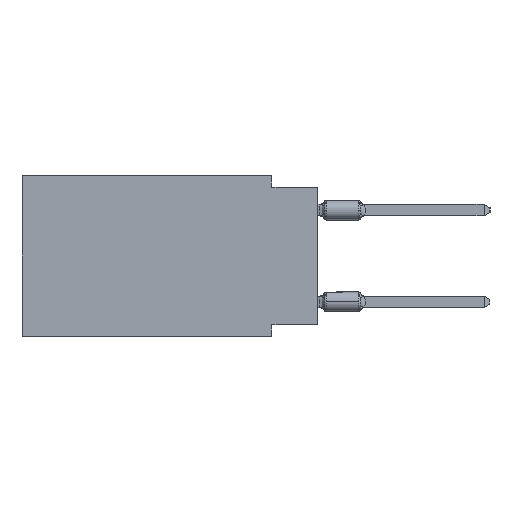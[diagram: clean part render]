
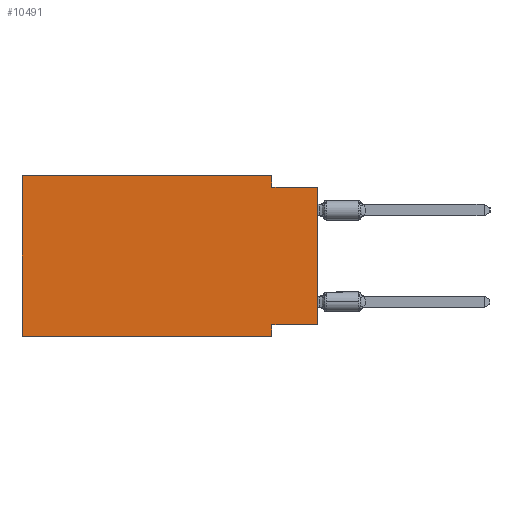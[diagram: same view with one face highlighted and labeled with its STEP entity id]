
A CAD part, left-side view. The second image highlights one B-rep face of the part: STEP entity #10491.
In plain terms, the highlighted planar face has unit normal (-1, 0, 0).
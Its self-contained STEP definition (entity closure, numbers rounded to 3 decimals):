
#1239 = CARTESIAN_POINT ( 'NONE',  ( 0., 16.383, 0. ) ) ;
#2220 = DIRECTION ( 'NONE',  ( 0., 0., 1. ) ) ;
#2269 = CARTESIAN_POINT ( 'NONE',  ( 0., 2.54, -0.635 ) ) ;
#2638 = ORIENTED_EDGE ( 'NONE', *, *, #15084, .T. ) ;
#2737 = LINE ( 'NONE', #10345, #23848 ) ;
#2896 = EDGE_CURVE ( 'NONE', #24381, #5201, #14568, .T. ) ;
#3232 = LINE ( 'NONE', #1239, #19793 ) ;
#3311 = CARTESIAN_POINT ( 'NONE',  ( 0., 0., -0.635 ) ) ;
#3857 = CARTESIAN_POINT ( 'NONE',  ( 0., 16.383, 0. ) ) ;
#4257 = EDGE_CURVE ( 'NONE', #8204, #5927, #3232, .T. ) ;
#4391 = EDGE_CURVE ( 'NONE', #21797, #8204, #22811, .T. ) ;
#4645 = VECTOR ( 'NONE', #2220, 1000. ) ;
#5201 = VERTEX_POINT ( 'NONE', #11739 ) ;
#5256 = PLANE ( 'NONE',  #18467 ) ;
#5927 = VERTEX_POINT ( 'NONE', #16566 ) ;
#5961 = CARTESIAN_POINT ( 'NONE',  ( 0., 0., 0. ) ) ;
#6499 = EDGE_CURVE ( 'NONE', #5201, #7645, #16034, .T. ) ;
#6882 = CARTESIAN_POINT ( 'NONE',  ( 0., 0., -0.635 ) ) ;
#7252 = CARTESIAN_POINT ( 'NONE',  ( 0., 16.383, 0. ) ) ;
#7645 = VERTEX_POINT ( 'NONE', #9715 ) ;
#7863 = ORIENTED_EDGE ( 'NONE', *, *, #6499, .F. ) ;
#7906 = EDGE_LOOP ( 'NONE', ( #2638, #11897, #16491, #15100, #22252, #21277, #7863, #11679 ) ) ;
#8204 = VERTEX_POINT ( 'NONE', #21805 ) ;
#8437 = VERTEX_POINT ( 'NONE', #2269 ) ;
#8915 = DIRECTION ( 'NONE',  ( 0., 0., -1. ) ) ;
#9715 = CARTESIAN_POINT ( 'NONE',  ( 0., 2.54, -8.89 ) ) ;
#10127 = DIRECTION ( 'NONE',  ( 0., 0., -1. ) ) ;
#10345 = CARTESIAN_POINT ( 'NONE',  ( 0., 16.383, -8.89 ) ) ;
#10491 = ADVANCED_FACE ( 'NONE', ( #11125 ), #5256, .F. ) ;
#10606 = DIRECTION ( 'NONE',  ( 0., -1., 0. ) ) ;
#10751 = DIRECTION ( 'NONE',  ( 1., 0., 0. ) ) ;
#11125 = FACE_OUTER_BOUND ( 'NONE', #7906, .T. ) ;
#11294 = CARTESIAN_POINT ( 'NONE',  ( 0., 0., -8.255 ) ) ;
#11679 = ORIENTED_EDGE ( 'NONE', *, *, #2896, .F. ) ;
#11739 = CARTESIAN_POINT ( 'NONE',  ( 0., 2.54, -8.255 ) ) ;
#11897 = ORIENTED_EDGE ( 'NONE', *, *, #16237, .F. ) ;
#13473 = VECTOR ( 'NONE', #8915, 1000. ) ;
#14568 = LINE ( 'NONE', #22060, #17123 ) ;
#15084 = EDGE_CURVE ( 'NONE', #24381, #21412, #15801, .T. ) ;
#15100 = ORIENTED_EDGE ( 'NONE', *, *, #4257, .F. ) ;
#15801 = LINE ( 'NONE', #5961, #16964 ) ;
#16034 = LINE ( 'NONE', #17924, #13473 ) ;
#16237 = EDGE_CURVE ( 'NONE', #8437, #21412, #20480, .T. ) ;
#16251 = CARTESIAN_POINT ( 'NONE',  ( 0., 2.54, 0. ) ) ;
#16491 = ORIENTED_EDGE ( 'NONE', *, *, #17323, .F. ) ;
#16566 = CARTESIAN_POINT ( 'NONE',  ( 0., 2.54, 0. ) ) ;
#16964 = VECTOR ( 'NONE', #23417, 1000. ) ;
#17123 = VECTOR ( 'NONE', #18191, 1000. ) ;
#17323 = EDGE_CURVE ( 'NONE', #5927, #8437, #23727, .T. ) ;
#17924 = CARTESIAN_POINT ( 'NONE',  ( 0., 2.54, -8.89 ) ) ;
#18191 = DIRECTION ( 'NONE',  ( 0., 1., 0. ) ) ;
#18467 = AXIS2_PLACEMENT_3D ( 'NONE', #7252, #10751, #22364 ) ;
#18587 = EDGE_CURVE ( 'NONE', #21797, #7645, #2737, .T. ) ;
#19377 = VECTOR ( 'NONE', #24342, 1000. ) ;
#19414 = VECTOR ( 'NONE', #10127, 1000. ) ;
#19793 = VECTOR ( 'NONE', #10606, 1000. ) ;
#20480 = LINE ( 'NONE', #6882, #19377 ) ;
#21277 = ORIENTED_EDGE ( 'NONE', *, *, #18587, .T. ) ;
#21412 = VERTEX_POINT ( 'NONE', #3311 ) ;
#21797 = VERTEX_POINT ( 'NONE', #24479 ) ;
#21805 = CARTESIAN_POINT ( 'NONE',  ( 0., 16.383, 0. ) ) ;
#21842 = DIRECTION ( 'NONE',  ( 0., -1., 0. ) ) ;
#22060 = CARTESIAN_POINT ( 'NONE',  ( 0., 0., -8.255 ) ) ;
#22252 = ORIENTED_EDGE ( 'NONE', *, *, #4391, .F. ) ;
#22364 = DIRECTION ( 'NONE',  ( 0., 0., -1. ) ) ;
#22811 = LINE ( 'NONE', #3857, #4645 ) ;
#23417 = DIRECTION ( 'NONE',  ( 0., 0., 1. ) ) ;
#23727 = LINE ( 'NONE', #16251, #19414 ) ;
#23848 = VECTOR ( 'NONE', #21842, 1000. ) ;
#24342 = DIRECTION ( 'NONE',  ( 0., -1., 0. ) ) ;
#24381 = VERTEX_POINT ( 'NONE', #11294 ) ;
#24479 = CARTESIAN_POINT ( 'NONE',  ( 0., 16.383, -8.89 ) ) ;
